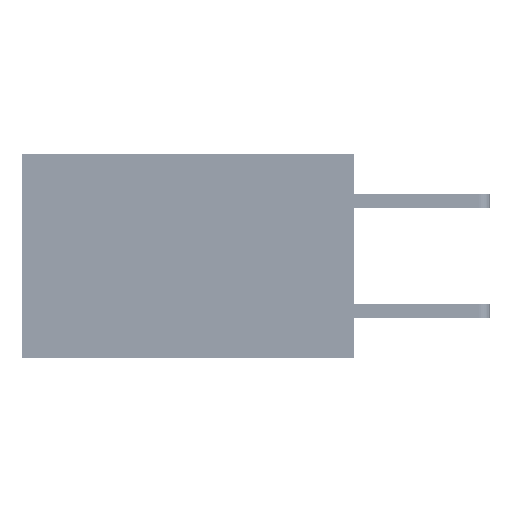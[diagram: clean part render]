
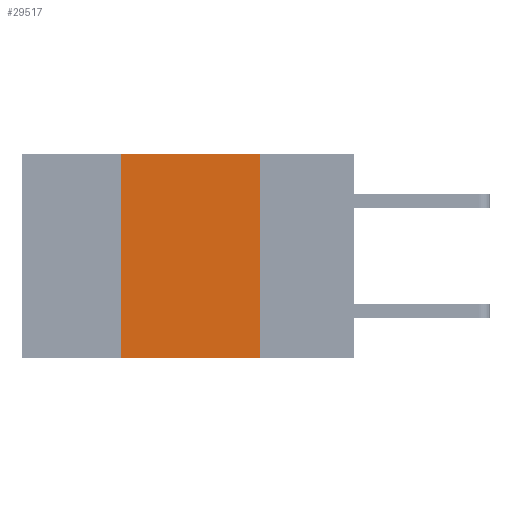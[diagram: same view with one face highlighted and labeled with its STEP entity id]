
A CAD part, left-side view. The second image highlights one B-rep face of the part: STEP entity #29517.
In plain terms, the highlighted planar face has unit normal (-1, 0, 0).
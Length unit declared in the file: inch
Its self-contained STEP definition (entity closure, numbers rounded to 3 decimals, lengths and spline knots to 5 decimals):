
#1031 = EDGE_CURVE ( 'NONE', #21728, #32689, #45336, .T. ) ;
#3850 = ORIENTED_EDGE ( 'NONE', *, *, #1031, .T. ) ;
#6099 = LINE ( 'NONE', #21154, #51135 ) ;
#8085 = LINE ( 'NONE', #40510, #9051 ) ;
#9051 = VECTOR ( 'NONE', #43899, 39.37008 ) ;
#9905 = EDGE_CURVE ( 'NONE', #40951, #32689, #8085, .T. ) ;
#10227 = VECTOR ( 'NONE', #38504, 39.37008 ) ;
#16038 = ORIENTED_EDGE ( 'NONE', *, *, #34167, .F. ) ;
#19970 = VECTOR ( 'NONE', #33978, 39.37008 ) ;
#21154 = CARTESIAN_POINT ( 'NONE',  ( 0., 0.6, 0. ) ) ;
#21728 = VERTEX_POINT ( 'NONE', #44815 ) ;
#22690 = CARTESIAN_POINT ( 'NONE',  ( 0., 0.6, -0.37 ) ) ;
#23252 = CARTESIAN_POINT ( 'NONE',  ( 0., 0.42, 0. ) ) ;
#26265 = CARTESIAN_POINT ( 'NONE',  ( 0., 0.42, 0. ) ) ;
#28999 = PLANE ( 'NONE',  #39657 ) ;
#29517 = ADVANCED_FACE ( 'NONE', ( #37562 ), #28999, .F. ) ;
#32689 = VERTEX_POINT ( 'NONE', #49468 ) ;
#33681 = DIRECTION ( 'NONE',  ( 0., 0., -1. ) ) ;
#33978 = DIRECTION ( 'NONE',  ( 0., 0., 1. ) ) ;
#34167 = EDGE_CURVE ( 'NONE', #21728, #40542, #45655, .T. ) ;
#36994 = ORIENTED_EDGE ( 'NONE', *, *, #9905, .F. ) ;
#37289 = DIRECTION ( 'NONE',  ( 1., 0., 0. ) ) ;
#37562 = FACE_OUTER_BOUND ( 'NONE', #45325, .T. ) ;
#38504 = DIRECTION ( 'NONE',  ( 0., -1., 0. ) ) ;
#38539 = EDGE_CURVE ( 'NONE', #40542, #40951, #6099, .T. ) ;
#39657 = AXIS2_PLACEMENT_3D ( 'NONE', #48464, #37289, #33681 ) ;
#40510 = CARTESIAN_POINT ( 'NONE',  ( 0., 0.17, 0. ) ) ;
#40542 = VERTEX_POINT ( 'NONE', #26265 ) ;
#40951 = VERTEX_POINT ( 'NONE', #45913 ) ;
#42685 = ORIENTED_EDGE ( 'NONE', *, *, #38539, .F. ) ;
#43899 = DIRECTION ( 'NONE',  ( 0., 0., -1. ) ) ;
#44815 = CARTESIAN_POINT ( 'NONE',  ( 0., 0.42, -0.37 ) ) ;
#45325 = EDGE_LOOP ( 'NONE', ( #36994, #42685, #16038, #3850 ) ) ;
#45336 = LINE ( 'NONE', #22690, #10227 ) ;
#45655 = LINE ( 'NONE', #23252, #19970 ) ;
#45913 = CARTESIAN_POINT ( 'NONE',  ( 0., 0.17, 0. ) ) ;
#48464 = CARTESIAN_POINT ( 'NONE',  ( 0., 0.6, 0. ) ) ;
#49468 = CARTESIAN_POINT ( 'NONE',  ( 0., 0.17, -0.37 ) ) ;
#49673 = DIRECTION ( 'NONE',  ( 0., -1., 0. ) ) ;
#51135 = VECTOR ( 'NONE', #49673, 39.37008 ) ;
